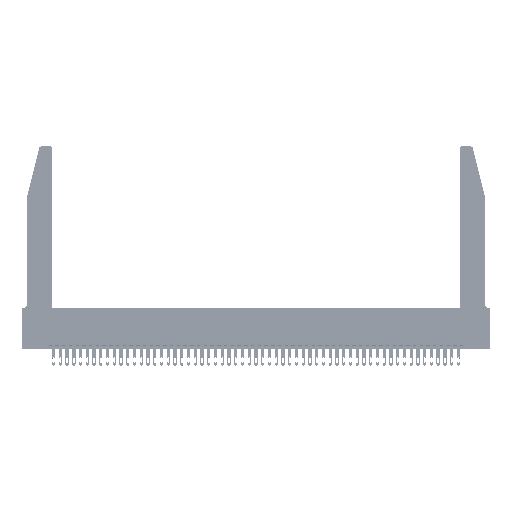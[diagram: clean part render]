
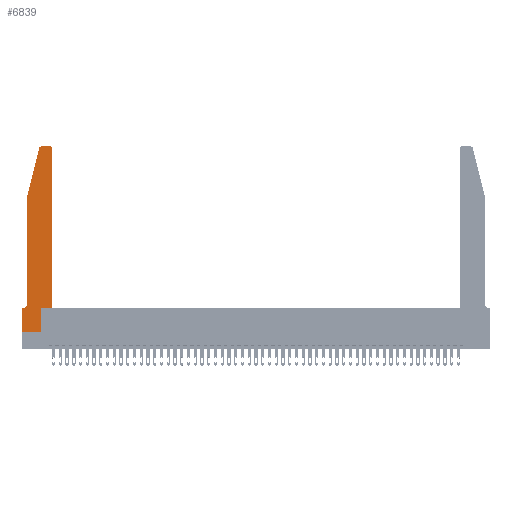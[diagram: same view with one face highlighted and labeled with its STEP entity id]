
A CAD part, top view. The second image highlights one B-rep face of the part: STEP entity #6839.
In plain terms, the highlighted planar face has unit normal (0, 0, 1).
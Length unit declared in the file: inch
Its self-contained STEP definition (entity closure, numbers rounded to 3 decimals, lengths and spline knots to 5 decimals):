
#525 = VERTEX_POINT ( 'NONE', #39771 ) ;
#643 = CARTESIAN_POINT ( 'NONE',  ( 0., 0.35, 0.37 ) ) ;
#800 = CARTESIAN_POINT ( 'NONE',  ( 0.4505, 0.35, 0.37 ) ) ;
#1579 = EDGE_CURVE ( 'NONE', #14996, #45682, #3632, .T. ) ;
#1588 = EDGE_CURVE ( 'NONE', #9240, #525, #6046, .T. ) ;
#1819 = ORIENTED_EDGE ( 'NONE', *, *, #10832, .T. ) ;
#2106 = LINE ( 'NONE', #35149, #17790 ) ;
#2421 = LINE ( 'NONE', #2892, #44071 ) ;
#2892 = CARTESIAN_POINT ( 'NONE',  ( 0., 0., 0.37 ) ) ;
#3632 = CIRCLE ( 'NONE', #28786, 0.07 ) ;
#4205 = VERTEX_POINT ( 'NONE', #800 ) ;
#4248 = DIRECTION ( 'NONE',  ( 1., 0., 0. ) ) ;
#5134 = CIRCLE ( 'NONE', #43712, 0.03 ) ;
#5970 = ORIENTED_EDGE ( 'NONE', *, *, #35350, .T. ) ;
#6046 = LINE ( 'NONE', #45284, #42334 ) ;
#6256 = VECTOR ( 'NONE', #34376, 39.37008 ) ;
#6263 = CARTESIAN_POINT ( 'NONE',  ( 0.2865, 0., 0.37 ) ) ;
#6540 = EDGE_CURVE ( 'NONE', #16452, #13369, #44111, .T. ) ;
#6569 = ORIENTED_EDGE ( 'NONE', *, *, #32536, .T. ) ;
#6839 = ADVANCED_FACE ( 'NONE', ( #18160 ), #40608, .T. ) ;
#6901 = CARTESIAN_POINT ( 'NONE',  ( 0.4505, 2.72, 0.37 ) ) ;
#7571 = DIRECTION ( 'NONE',  ( -0.239, -0.971, 0. ) ) ;
#7780 = DIRECTION ( 'NONE',  ( 1., 0., 0. ) ) ;
#8069 = ORIENTED_EDGE ( 'NONE', *, *, #15355, .T. ) ;
#8264 = LINE ( 'NONE', #46338, #43949 ) ;
#9240 = VERTEX_POINT ( 'NONE', #6263 ) ;
#9846 = DIRECTION ( 'NONE',  ( 0., 0., 1. ) ) ;
#10162 = DIRECTION ( 'NONE',  ( 0., -1., 0. ) ) ;
#10832 = EDGE_CURVE ( 'NONE', #4205, #10971, #44440, .T. ) ;
#10971 = VERTEX_POINT ( 'NONE', #6901 ) ;
#11206 = DIRECTION ( 'NONE',  ( 0., 0., 1. ) ) ;
#13141 = EDGE_CURVE ( 'NONE', #13369, #25746, #30327, .T. ) ;
#13236 = CARTESIAN_POINT ( 'NONE',  ( 0., 0.35, 0.37 ) ) ;
#13369 = VERTEX_POINT ( 'NONE', #39056 ) ;
#13988 = CARTESIAN_POINT ( 'NONE',  ( 0.0055, 0.42, 0.37 ) ) ;
#14996 = VERTEX_POINT ( 'NONE', #30630 ) ;
#15355 = EDGE_CURVE ( 'NONE', #45682, #17719, #48635, .T. ) ;
#16452 = VERTEX_POINT ( 'NONE', #24859 ) ;
#16700 = EDGE_LOOP ( 'NONE', ( #47755, #23294, #47600, #24012, #26143, #8069, #31856, #17234, #21021, #5970, #1819, #6569 ) ) ;
#17175 = VECTOR ( 'NONE', #40879, 39.37008 ) ;
#17234 = ORIENTED_EDGE ( 'NONE', *, *, #40058, .T. ) ;
#17255 = DIRECTION ( 'NONE',  ( 1., 0., 0. ) ) ;
#17688 = CARTESIAN_POINT ( 'NONE',  ( 0.0755, 0.35, 0.37 ) ) ;
#17719 = VERTEX_POINT ( 'NONE', #643 ) ;
#17790 = VECTOR ( 'NONE', #7780, 39.37008 ) ;
#17833 = DIRECTION ( 'NONE',  ( 0., 1., 0. ) ) ;
#17856 = DIRECTION ( 'NONE',  ( 0., 0., -1. ) ) ;
#17999 = VERTEX_POINT ( 'NONE', #34069 ) ;
#18160 = FACE_OUTER_BOUND ( 'NONE', #16700, .T. ) ;
#18764 = CARTESIAN_POINT ( 'NONE',  ( 0.2605, 2.75, 0.37 ) ) ;
#19699 = CARTESIAN_POINT ( 'NONE',  ( 0.0755, 2., 0.37 ) ) ;
#20833 = DIRECTION ( 'NONE',  ( 1., 0., 0. ) ) ;
#21021 = ORIENTED_EDGE ( 'NONE', *, *, #1588, .T. ) ;
#21773 = LINE ( 'NONE', #19699, #33906 ) ;
#21940 = EDGE_CURVE ( 'NONE', #45965, #14996, #49167, .T. ) ;
#22811 = CARTESIAN_POINT ( 'NONE',  ( 0.284, 2.72, 0.37 ) ) ;
#23294 = ORIENTED_EDGE ( 'NONE', *, *, #13141, .T. ) ;
#23387 = EDGE_CURVE ( 'NONE', #25746, #45965, #21773, .T. ) ;
#24012 = ORIENTED_EDGE ( 'NONE', *, *, #21940, .T. ) ;
#24450 = EDGE_CURVE ( 'NONE', #17719, #17999, #2421, .T. ) ;
#24859 = CARTESIAN_POINT ( 'NONE',  ( 0.4205, 2.75, 0.37 ) ) ;
#25746 = VERTEX_POINT ( 'NONE', #41521 ) ;
#25813 = AXIS2_PLACEMENT_3D ( 'NONE', #13236, #48058, #17255 ) ;
#25820 = DIRECTION ( 'NONE',  ( 0., 1., 0. ) ) ;
#26143 = ORIENTED_EDGE ( 'NONE', *, *, #1579, .T. ) ;
#26904 = DIRECTION ( 'NONE',  ( 1., 0., 0. ) ) ;
#28786 = AXIS2_PLACEMENT_3D ( 'NONE', #13988, #17856, #44944 ) ;
#30327 = CIRCLE ( 'NONE', #40851, 0.03 ) ;
#30630 = CARTESIAN_POINT ( 'NONE',  ( 0.0755, 0.42, 0.37 ) ) ;
#31856 = ORIENTED_EDGE ( 'NONE', *, *, #24450, .T. ) ;
#32536 = EDGE_CURVE ( 'NONE', #10971, #16452, #5134, .T. ) ;
#33011 = CARTESIAN_POINT ( 'NONE',  ( 0.4205, 2.72, 0.37 ) ) ;
#33405 = CARTESIAN_POINT ( 'NONE',  ( 0.4505, 0.35, 0.37 ) ) ;
#33906 = VECTOR ( 'NONE', #7571, 39.37008 ) ;
#34069 = CARTESIAN_POINT ( 'NONE',  ( 0., 0., 0.37 ) ) ;
#34376 = DIRECTION ( 'NONE',  ( 0., -1., 0. ) ) ;
#34707 = CARTESIAN_POINT ( 'NONE',  ( 0.0755, 2., 0.37 ) ) ;
#35149 = CARTESIAN_POINT ( 'NONE',  ( 0.4505, 0.35, 0.37 ) ) ;
#35350 = EDGE_CURVE ( 'NONE', #525, #4205, #2106, .T. ) ;
#37189 = VECTOR ( 'NONE', #17833, 39.37008 ) ;
#39056 = CARTESIAN_POINT ( 'NONE',  ( 0.284, 2.75, 0.37 ) ) ;
#39771 = CARTESIAN_POINT ( 'NONE',  ( 0.2865, 0.35, 0.37 ) ) ;
#39855 = DIRECTION ( 'NONE',  ( -1., 0., 0. ) ) ;
#40058 = EDGE_CURVE ( 'NONE', #17999, #9240, #8264, .T. ) ;
#40608 = PLANE ( 'NONE',  #25813 ) ;
#40851 = AXIS2_PLACEMENT_3D ( 'NONE', #22811, #11206, #26904 ) ;
#40879 = DIRECTION ( 'NONE',  ( -1., 0., 0. ) ) ;
#41521 = CARTESIAN_POINT ( 'NONE',  ( 0.25487, 2.72718, 0.37 ) ) ;
#42334 = VECTOR ( 'NONE', #25820, 39.37008 ) ;
#43712 = AXIS2_PLACEMENT_3D ( 'NONE', #33011, #9846, #20833 ) ;
#43949 = VECTOR ( 'NONE', #4248, 39.37008 ) ;
#44071 = VECTOR ( 'NONE', #10162, 39.37008 ) ;
#44111 = LINE ( 'NONE', #18764, #48912 ) ;
#44339 = CARTESIAN_POINT ( 'NONE',  ( 0.0755, 2., 0.37 ) ) ;
#44440 = LINE ( 'NONE', #33405, #37189 ) ;
#44944 = DIRECTION ( 'NONE',  ( -1., 0., 0. ) ) ;
#45284 = CARTESIAN_POINT ( 'NONE',  ( 0.2865, 0.35, 0.37 ) ) ;
#45682 = VERTEX_POINT ( 'NONE', #49957 ) ;
#45965 = VERTEX_POINT ( 'NONE', #44339 ) ;
#46338 = CARTESIAN_POINT ( 'NONE',  ( 0., 0., 0.37 ) ) ;
#47600 = ORIENTED_EDGE ( 'NONE', *, *, #23387, .T. ) ;
#47755 = ORIENTED_EDGE ( 'NONE', *, *, #6540, .T. ) ;
#48058 = DIRECTION ( 'NONE',  ( 0., 0., 1. ) ) ;
#48635 = LINE ( 'NONE', #17688, #17175 ) ;
#48912 = VECTOR ( 'NONE', #39855, 39.37008 ) ;
#49167 = LINE ( 'NONE', #34707, #6256 ) ;
#49957 = CARTESIAN_POINT ( 'NONE',  ( 0.0055, 0.35, 0.37 ) ) ;
